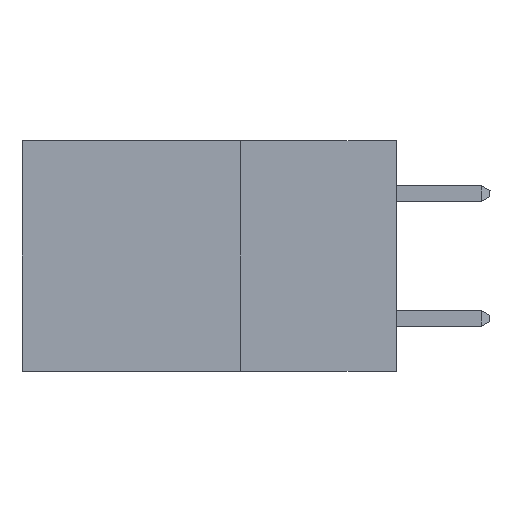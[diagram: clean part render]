
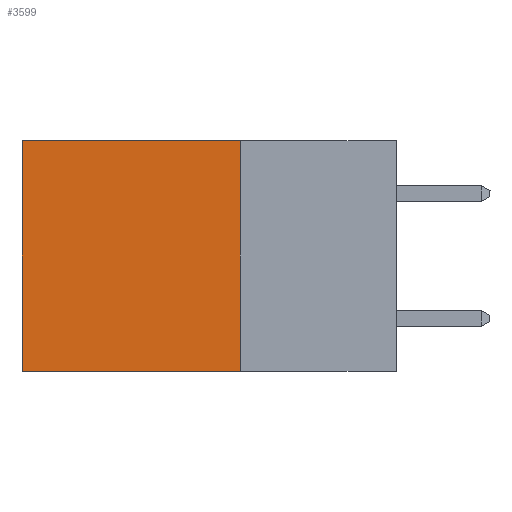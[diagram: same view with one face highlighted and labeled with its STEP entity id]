
A CAD part, left-side view. The second image highlights one B-rep face of the part: STEP entity #3599.
In plain terms, the highlighted planar face has unit normal (-1, 0, 0).
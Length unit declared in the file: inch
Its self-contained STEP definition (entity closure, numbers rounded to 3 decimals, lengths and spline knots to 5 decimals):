
#91 = LINE ( 'NONE', #12039, #8318 ) ;
#277 = ORIENTED_EDGE ( 'NONE', *, *, #11212, .F. ) ;
#348 = CARTESIAN_POINT ( 'NONE',  ( 0.298, 0.25, 0. ) ) ;
#1204 = CARTESIAN_POINT ( 'NONE',  ( 0.298, 0.25, -0.37 ) ) ;
#1291 = PLANE ( 'NONE',  #6333 ) ;
#1811 = EDGE_CURVE ( 'NONE', #11321, #10915, #91, .T. ) ;
#2076 = ORIENTED_EDGE ( 'NONE', *, *, #8993, .F. ) ;
#3312 = FACE_OUTER_BOUND ( 'NONE', #13601, .T. ) ;
#3426 = VECTOR ( 'NONE', #12682, 39.37008 ) ;
#3599 = ADVANCED_FACE ( 'NONE', ( #3312 ), #1291, .F. ) ;
#4193 = CARTESIAN_POINT ( 'NONE',  ( 0.298, 0.6, 0. ) ) ;
#4248 = DIRECTION ( 'NONE',  ( 1., 0., 0. ) ) ;
#5777 = CARTESIAN_POINT ( 'NONE',  ( 0.298, 0.6, -0.37 ) ) ;
#5904 = LINE ( 'NONE', #4193, #3426 ) ;
#6224 = EDGE_CURVE ( 'NONE', #10915, #9352, #5904, .T. ) ;
#6325 = CARTESIAN_POINT ( 'NONE',  ( 0.298, 0.6, 0. ) ) ;
#6333 = AXIS2_PLACEMENT_3D ( 'NONE', #13445, #4248, #11554 ) ;
#6926 = ORIENTED_EDGE ( 'NONE', *, *, #6224, .T. ) ;
#7074 = DIRECTION ( 'NONE',  ( 0., 1., 0. ) ) ;
#7873 = DIRECTION ( 'NONE',  ( 0., 0., -1. ) ) ;
#8046 = CARTESIAN_POINT ( 'NONE',  ( 0.298, 0.25, 0. ) ) ;
#8318 = VECTOR ( 'NONE', #7074, 39.37008 ) ;
#8619 = ORIENTED_EDGE ( 'NONE', *, *, #1811, .T. ) ;
#8993 = EDGE_CURVE ( 'NONE', #9188, #9352, #10225, .T. ) ;
#9188 = VERTEX_POINT ( 'NONE', #1204 ) ;
#9352 = VERTEX_POINT ( 'NONE', #5777 ) ;
#9502 = VECTOR ( 'NONE', #7873, 39.37008 ) ;
#10225 = LINE ( 'NONE', #10421, #12463 ) ;
#10421 = CARTESIAN_POINT ( 'NONE',  ( 0.298, 0.25, -0.37 ) ) ;
#10915 = VERTEX_POINT ( 'NONE', #6325 ) ;
#11212 = EDGE_CURVE ( 'NONE', #11321, #9188, #12396, .T. ) ;
#11321 = VERTEX_POINT ( 'NONE', #8046 ) ;
#11530 = DIRECTION ( 'NONE',  ( 0., 1., 0. ) ) ;
#11554 = DIRECTION ( 'NONE',  ( 0., 0., -1. ) ) ;
#12039 = CARTESIAN_POINT ( 'NONE',  ( 0.298, 0.25, 0. ) ) ;
#12396 = LINE ( 'NONE', #348, #9502 ) ;
#12463 = VECTOR ( 'NONE', #11530, 39.37008 ) ;
#12682 = DIRECTION ( 'NONE',  ( 0., 0., -1. ) ) ;
#13445 = CARTESIAN_POINT ( 'NONE',  ( 0.298, 0.25, 0. ) ) ;
#13601 = EDGE_LOOP ( 'NONE', ( #6926, #2076, #277, #8619 ) ) ;
